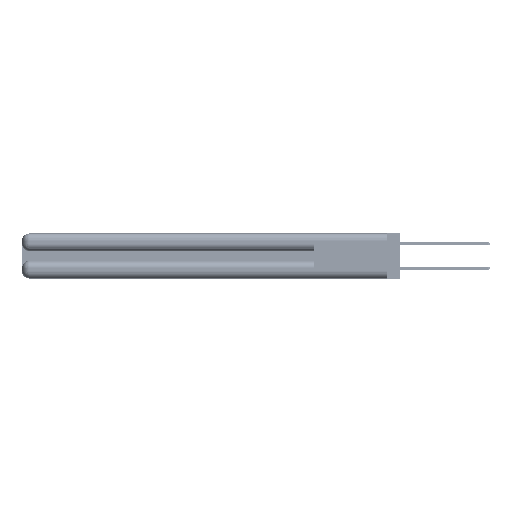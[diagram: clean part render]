
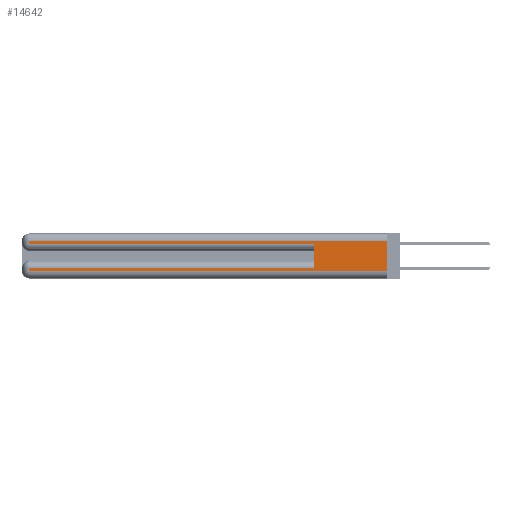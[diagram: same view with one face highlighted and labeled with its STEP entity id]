
A CAD part, left-side view. The second image highlights one B-rep face of the part: STEP entity #14642.
In plain terms, the highlighted planar face has unit normal (-1, 0, 0).
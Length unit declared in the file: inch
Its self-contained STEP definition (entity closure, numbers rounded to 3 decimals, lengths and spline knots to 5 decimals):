
#431 = VECTOR ( 'NONE', #10311, 39.37008 ) ;
#4171 = ORIENTED_EDGE ( 'NONE', *, *, #27885, .T. ) ;
#4291 = DIRECTION ( 'NONE',  ( 0., 0., -1. ) ) ;
#6329 = LINE ( 'NONE', #14163, #431 ) ;
#7081 = EDGE_CURVE ( 'NONE', #51420, #9377, #17362, .T. ) ;
#8147 = EDGE_CURVE ( 'NONE', #39888, #20416, #13971, .T. ) ;
#8290 = EDGE_CURVE ( 'NONE', #38878, #12143, #49390, .T. ) ;
#9377 = VERTEX_POINT ( 'NONE', #24305 ) ;
#10273 = VECTOR ( 'NONE', #26849, 39.37008 ) ;
#10311 = DIRECTION ( 'NONE',  ( 0., 1., 0. ) ) ;
#10392 = EDGE_CURVE ( 'NONE', #38878, #39888, #6329, .T. ) ;
#10537 = CARTESIAN_POINT ( 'NONE',  ( 0., 0.6, 0.085 ) ) ;
#11039 = CARTESIAN_POINT ( 'NONE',  ( 0., 2.94, 0.06 ) ) ;
#11473 = VECTOR ( 'NONE', #4291, 39.37008 ) ;
#12143 = VERTEX_POINT ( 'NONE', #41935 ) ;
#13274 = EDGE_CURVE ( 'NONE', #20416, #32238, #34075, .T. ) ;
#13971 = LINE ( 'NONE', #27954, #48119 ) ;
#14163 = CARTESIAN_POINT ( 'NONE',  ( 0., 0., 0.085 ) ) ;
#14642 = ADVANCED_FACE ( 'NONE', ( #18241 ), #35351, .F. ) ;
#14835 = LINE ( 'NONE', #51999, #10273 ) ;
#16658 = DIRECTION ( 'NONE',  ( 0., -1., 0. ) ) ;
#17362 = LINE ( 'NONE', #51656, #19317 ) ;
#17853 = VECTOR ( 'NONE', #37409, 39.37008 ) ;
#18241 = FACE_OUTER_BOUND ( 'NONE', #37110, .T. ) ;
#19317 = VECTOR ( 'NONE', #26682, 39.37008 ) ;
#20039 = ORIENTED_EDGE ( 'NONE', *, *, #8290, .F. ) ;
#20053 = DIRECTION ( 'NONE',  ( 0., 0., -1. ) ) ;
#20416 = VERTEX_POINT ( 'NONE', #11039 ) ;
#20878 = VECTOR ( 'NONE', #32868, 39.37008 ) ;
#22343 = CARTESIAN_POINT ( 'NONE',  ( 0., 0., 0.06 ) ) ;
#22643 = CARTESIAN_POINT ( 'NONE',  ( 0., 0., 0.31 ) ) ;
#24119 = CARTESIAN_POINT ( 'NONE',  ( 0., 0., 0.285 ) ) ;
#24305 = CARTESIAN_POINT ( 'NONE',  ( 0., 2.94, 0.31 ) ) ;
#24822 = CARTESIAN_POINT ( 'NONE',  ( 0., 0.6, 0.145 ) ) ;
#25677 = VERTEX_POINT ( 'NONE', #49245 ) ;
#25694 = ORIENTED_EDGE ( 'NONE', *, *, #38994, .F. ) ;
#26682 = DIRECTION ( 'NONE',  ( 0., 1., 0. ) ) ;
#26849 = DIRECTION ( 'NONE',  ( 0., 0., -1. ) ) ;
#27885 = EDGE_CURVE ( 'NONE', #9377, #25677, #36952, .T. ) ;
#27954 = CARTESIAN_POINT ( 'NONE',  ( 0., 2.94, 0.37 ) ) ;
#29393 = CARTESIAN_POINT ( 'NONE',  ( 0., 2.94, 0.37 ) ) ;
#30985 = DIRECTION ( 'NONE',  ( 1., 0., 0. ) ) ;
#31864 = CARTESIAN_POINT ( 'NONE',  ( 0., 0., 0.06 ) ) ;
#32238 = VERTEX_POINT ( 'NONE', #31864 ) ;
#32759 = ORIENTED_EDGE ( 'NONE', *, *, #48654, .T. ) ;
#32868 = DIRECTION ( 'NONE',  ( 0., -1., 0. ) ) ;
#34065 = CARTESIAN_POINT ( 'NONE',  ( 0., 2.94, 0.085 ) ) ;
#34075 = LINE ( 'NONE', #22343, #35399 ) ;
#34815 = DIRECTION ( 'NONE',  ( 0., 0., -1. ) ) ;
#35351 = PLANE ( 'NONE',  #35916 ) ;
#35399 = VECTOR ( 'NONE', #16658, 39.37008 ) ;
#35916 = AXIS2_PLACEMENT_3D ( 'NONE', #42859, #30985, #34815 ) ;
#36952 = LINE ( 'NONE', #29393, #11473 ) ;
#37110 = EDGE_LOOP ( 'NONE', ( #25694, #44993, #4171, #32759, #20039, #41374, #49547, #45409 ) ) ;
#37409 = DIRECTION ( 'NONE',  ( 0., 0., 1. ) ) ;
#38878 = VERTEX_POINT ( 'NONE', #10537 ) ;
#38994 = EDGE_CURVE ( 'NONE', #51420, #32238, #14835, .T. ) ;
#39888 = VERTEX_POINT ( 'NONE', #34065 ) ;
#40481 = LINE ( 'NONE', #24119, #20878 ) ;
#41374 = ORIENTED_EDGE ( 'NONE', *, *, #10392, .T. ) ;
#41935 = CARTESIAN_POINT ( 'NONE',  ( 0., 0.6, 0.285 ) ) ;
#42859 = CARTESIAN_POINT ( 'NONE',  ( 0., 0., 0.37 ) ) ;
#44993 = ORIENTED_EDGE ( 'NONE', *, *, #7081, .T. ) ;
#45409 = ORIENTED_EDGE ( 'NONE', *, *, #13274, .T. ) ;
#48119 = VECTOR ( 'NONE', #20053, 39.37008 ) ;
#48654 = EDGE_CURVE ( 'NONE', #25677, #12143, #40481, .T. ) ;
#49245 = CARTESIAN_POINT ( 'NONE',  ( 0., 2.94, 0.285 ) ) ;
#49390 = LINE ( 'NONE', #24822, #17853 ) ;
#49547 = ORIENTED_EDGE ( 'NONE', *, *, #8147, .T. ) ;
#51420 = VERTEX_POINT ( 'NONE', #22643 ) ;
#51656 = CARTESIAN_POINT ( 'NONE',  ( 0., 0., 0.31 ) ) ;
#51999 = CARTESIAN_POINT ( 'NONE',  ( 0., 0., 0.37 ) ) ;
